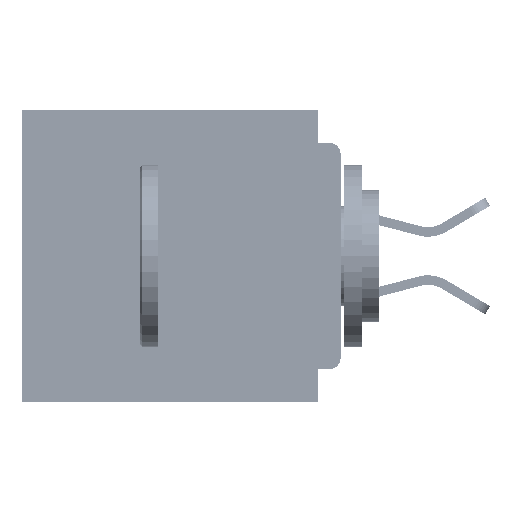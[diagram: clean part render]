
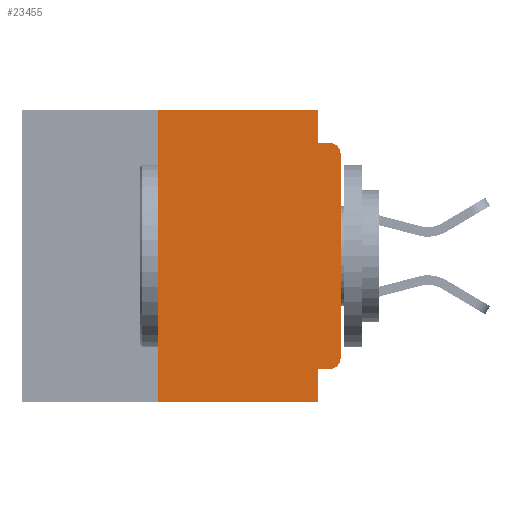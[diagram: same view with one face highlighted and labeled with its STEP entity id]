
A CAD part, left-side view. The second image highlights one B-rep face of the part: STEP entity #23455.
In plain terms, the highlighted planar face has unit normal (-1, 0, 0).
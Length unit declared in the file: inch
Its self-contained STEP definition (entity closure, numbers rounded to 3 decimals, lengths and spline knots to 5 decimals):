
#1597 = DIRECTION ( 'NONE',  ( 0., 0., 1. ) ) ;
#3250 = CARTESIAN_POINT ( 'NONE',  ( 0., 0.015, -0.355 ) ) ;
#5198 = DIRECTION ( 'NONE',  ( 0., 0., -1. ) ) ;
#5404 = CARTESIAN_POINT ( 'NONE',  ( 0., 0., -0.06 ) ) ;
#5595 = EDGE_CURVE ( 'NONE', #45547, #28781, #23010, .T. ) ;
#6557 = DIRECTION ( 'NONE',  ( 0., -1., 0. ) ) ;
#7121 = VERTEX_POINT ( 'NONE', #31149 ) ;
#7481 = PLANE ( 'NONE',  #32960 ) ;
#9363 = LINE ( 'NONE', #33472, #20568 ) ;
#10258 = VECTOR ( 'NONE', #5198, 39.37008 ) ;
#12917 = CARTESIAN_POINT ( 'NONE',  ( 0., 0., 0. ) ) ;
#13508 = CARTESIAN_POINT ( 'NONE',  ( 0., 0., -0.045 ) ) ;
#13564 = CARTESIAN_POINT ( 'NONE',  ( 0., 0.015, -0.06 ) ) ;
#15720 = ORIENTED_EDGE ( 'NONE', *, *, #49659, .F. ) ;
#15738 = EDGE_CURVE ( 'NONE', #7121, #22701, #19675, .T. ) ;
#16325 = ORIENTED_EDGE ( 'NONE', *, *, #25933, .F. ) ;
#17963 = ORIENTED_EDGE ( 'NONE', *, *, #45294, .T. ) ;
#18335 = DIRECTION ( 'NONE',  ( 0., -1., 0. ) ) ;
#18386 = DIRECTION ( 'NONE',  ( 0., 0., -1. ) ) ;
#19159 = CARTESIAN_POINT ( 'NONE',  ( 0., 0.015, -0.34 ) ) ;
#19214 = VERTEX_POINT ( 'NONE', #48796 ) ;
#19675 = LINE ( 'NONE', #30357, #59378 ) ;
#20568 = VECTOR ( 'NONE', #57511, 39.37008 ) ;
#21940 = CARTESIAN_POINT ( 'NONE',  ( 0., 0.437, 0. ) ) ;
#22275 = VECTOR ( 'NONE', #18335, 39.37008 ) ;
#22335 = VERTEX_POINT ( 'NONE', #32124 ) ;
#22535 = ORIENTED_EDGE ( 'NONE', *, *, #26164, .F. ) ;
#22701 = VERTEX_POINT ( 'NONE', #58654 ) ;
#23010 = LINE ( 'NONE', #12917, #47025 ) ;
#23455 = ADVANCED_FACE ( 'NONE', ( #45656 ), #7481, .F. ) ;
#24001 = DIRECTION ( 'NONE',  ( 0., 0., -1. ) ) ;
#24389 = CARTESIAN_POINT ( 'NONE',  ( 0., 0.031, -0.4 ) ) ;
#24980 = VECTOR ( 'NONE', #60957, 39.37008 ) ;
#25933 = EDGE_CURVE ( 'NONE', #22701, #19214, #27267, .T. ) ;
#26164 = EDGE_CURVE ( 'NONE', #27086, #47286, #61663, .T. ) ;
#26768 = DIRECTION ( 'NONE',  ( 0., 0., -1. ) ) ;
#27086 = VERTEX_POINT ( 'NONE', #35232 ) ;
#27267 = LINE ( 'NONE', #30481, #49805 ) ;
#27491 = CARTESIAN_POINT ( 'NONE',  ( 0., 0.031, -0.4 ) ) ;
#28028 = ORIENTED_EDGE ( 'NONE', *, *, #36678, .T. ) ;
#28781 = VERTEX_POINT ( 'NONE', #5404 ) ;
#29231 = CIRCLE ( 'NONE', #58337, 0.015 ) ;
#30357 = CARTESIAN_POINT ( 'NONE',  ( 0., 0.25, -0.4 ) ) ;
#30481 = CARTESIAN_POINT ( 'NONE',  ( 0., 0.437, 0. ) ) ;
#31149 = CARTESIAN_POINT ( 'NONE',  ( 0., 0.25, -0.4 ) ) ;
#31325 = VERTEX_POINT ( 'NONE', #56749 ) ;
#32124 = CARTESIAN_POINT ( 'NONE',  ( 0., 0.031, -0.045 ) ) ;
#32960 = AXIS2_PLACEMENT_3D ( 'NONE', #21940, #55476, #26768 ) ;
#33264 = ORIENTED_EDGE ( 'NONE', *, *, #52406, .F. ) ;
#33472 = CARTESIAN_POINT ( 'NONE',  ( 0., 0.437, -0.4 ) ) ;
#33880 = EDGE_CURVE ( 'NONE', #39347, #27086, #50540, .T. ) ;
#35093 = LINE ( 'NONE', #13508, #22275 ) ;
#35232 = CARTESIAN_POINT ( 'NONE',  ( 0., 0.031, -0.355 ) ) ;
#36678 = EDGE_CURVE ( 'NONE', #39347, #45547, #29231, .T. ) ;
#37037 = DIRECTION ( 'NONE',  ( 0., 1., 0. ) ) ;
#37327 = LINE ( 'NONE', #48403, #10258 ) ;
#37835 = EDGE_CURVE ( 'NONE', #28781, #31325, #50852, .T. ) ;
#39347 = VERTEX_POINT ( 'NONE', #3250 ) ;
#44986 = CARTESIAN_POINT ( 'NONE',  ( 0., 0., -0.34 ) ) ;
#45294 = EDGE_CURVE ( 'NONE', #7121, #47286, #9363, .T. ) ;
#45536 = EDGE_LOOP ( 'NONE', ( #60742, #60873, #33264, #15720, #16325, #55047, #17963, #22535, #62049, #28028 ) ) ;
#45547 = VERTEX_POINT ( 'NONE', #44986 ) ;
#45656 = FACE_OUTER_BOUND ( 'NONE', #45536, .T. ) ;
#46493 = DIRECTION ( 'NONE',  ( 0., 0., 1. ) ) ;
#47025 = VECTOR ( 'NONE', #46493, 39.37008 ) ;
#47141 = DIRECTION ( 'NONE',  ( -1., 0., 0. ) ) ;
#47286 = VERTEX_POINT ( 'NONE', #24389 ) ;
#48403 = CARTESIAN_POINT ( 'NONE',  ( 0., 0.031, 0. ) ) ;
#48796 = CARTESIAN_POINT ( 'NONE',  ( 0., 0.031, 0. ) ) ;
#49029 = VECTOR ( 'NONE', #37037, 39.37008 ) ;
#49659 = EDGE_CURVE ( 'NONE', #19214, #22335, #37327, .T. ) ;
#49805 = VECTOR ( 'NONE', #6557, 39.37008 ) ;
#50540 = LINE ( 'NONE', #56052, #49029 ) ;
#50852 = CIRCLE ( 'NONE', #53601, 0.015 ) ;
#52406 = EDGE_CURVE ( 'NONE', #22335, #31325, #35093, .T. ) ;
#52726 = DIRECTION ( 'NONE',  ( -1., 0., 0. ) ) ;
#53601 = AXIS2_PLACEMENT_3D ( 'NONE', #13564, #47141, #18386 ) ;
#55047 = ORIENTED_EDGE ( 'NONE', *, *, #15738, .F. ) ;
#55476 = DIRECTION ( 'NONE',  ( 1., 0., 0. ) ) ;
#56052 = CARTESIAN_POINT ( 'NONE',  ( 0., 0., -0.355 ) ) ;
#56749 = CARTESIAN_POINT ( 'NONE',  ( 0., 0.015, -0.045 ) ) ;
#57511 = DIRECTION ( 'NONE',  ( 0., -1., 0. ) ) ;
#58337 = AXIS2_PLACEMENT_3D ( 'NONE', #19159, #52726, #24001 ) ;
#58654 = CARTESIAN_POINT ( 'NONE',  ( 0., 0.25, 0. ) ) ;
#59378 = VECTOR ( 'NONE', #1597, 39.37008 ) ;
#60742 = ORIENTED_EDGE ( 'NONE', *, *, #5595, .T. ) ;
#60873 = ORIENTED_EDGE ( 'NONE', *, *, #37835, .T. ) ;
#60957 = DIRECTION ( 'NONE',  ( 0., 0., -1. ) ) ;
#61663 = LINE ( 'NONE', #27491, #24980 ) ;
#62049 = ORIENTED_EDGE ( 'NONE', *, *, #33880, .F. ) ;
